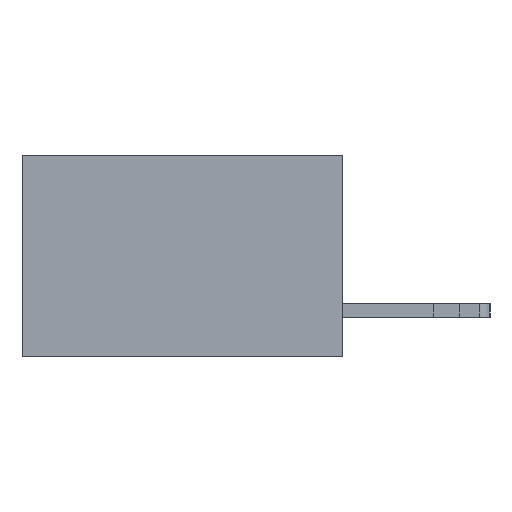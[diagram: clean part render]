
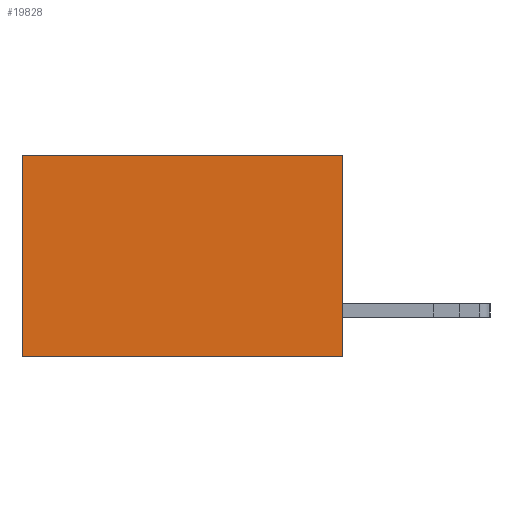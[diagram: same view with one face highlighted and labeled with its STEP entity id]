
A CAD part, left-side view. The second image highlights one B-rep face of the part: STEP entity #19828.
In plain terms, the highlighted planar face has unit normal (-1, 0, 0).
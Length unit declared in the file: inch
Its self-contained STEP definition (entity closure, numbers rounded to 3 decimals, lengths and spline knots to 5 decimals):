
#372 = VECTOR ( 'NONE', #17685, 39.37008 ) ;
#527 = EDGE_CURVE ( 'NONE', #11427, #15014, #13716, .T. ) ;
#1280 = DIRECTION ( 'NONE',  ( 0., 0., -1. ) ) ;
#1455 = CARTESIAN_POINT ( 'NONE',  ( 0.277, 0.59, -0.37 ) ) ;
#3148 = FACE_OUTER_BOUND ( 'NONE', #8072, .T. ) ;
#3642 = CARTESIAN_POINT ( 'NONE',  ( 0.277, 0., -0.37 ) ) ;
#3850 = ORIENTED_EDGE ( 'NONE', *, *, #6209, .F. ) ;
#4385 = CARTESIAN_POINT ( 'NONE',  ( 0.277, 0., 0. ) ) ;
#4778 = DIRECTION ( 'NONE',  ( 0., 0., -1. ) ) ;
#6189 = CARTESIAN_POINT ( 'NONE',  ( 0.277, 0., -0.37 ) ) ;
#6209 = EDGE_CURVE ( 'NONE', #8559, #17614, #8364, .T. ) ;
#6595 = CARTESIAN_POINT ( 'NONE',  ( 0.277, 0., -0.37 ) ) ;
#6766 = ORIENTED_EDGE ( 'NONE', *, *, #9300, .T. ) ;
#7045 = CARTESIAN_POINT ( 'NONE',  ( 0.277, 0., 0. ) ) ;
#7113 = VECTOR ( 'NONE', #8768, 39.37008 ) ;
#8072 = EDGE_LOOP ( 'NONE', ( #13944, #15072, #3850, #6766 ) ) ;
#8364 = LINE ( 'NONE', #6595, #12416 ) ;
#8559 = VERTEX_POINT ( 'NONE', #4385 ) ;
#8669 = CARTESIAN_POINT ( 'NONE',  ( 0.277, 0.59, -0.37 ) ) ;
#8768 = DIRECTION ( 'NONE',  ( 0., 1., 0. ) ) ;
#9300 = EDGE_CURVE ( 'NONE', #8559, #11427, #11163, .T. ) ;
#11163 = LINE ( 'NONE', #7045, #7113 ) ;
#11427 = VERTEX_POINT ( 'NONE', #17562 ) ;
#11622 = PLANE ( 'NONE',  #17821 ) ;
#12416 = VECTOR ( 'NONE', #1280, 39.37008 ) ;
#13359 = CARTESIAN_POINT ( 'NONE',  ( 0.277, 0., -0.37 ) ) ;
#13716 = LINE ( 'NONE', #1455, #372 ) ;
#13944 = ORIENTED_EDGE ( 'NONE', *, *, #527, .T. ) ;
#15014 = VERTEX_POINT ( 'NONE', #8669 ) ;
#15072 = ORIENTED_EDGE ( 'NONE', *, *, #15361, .F. ) ;
#15087 = DIRECTION ( 'NONE',  ( 1., 0., 0. ) ) ;
#15361 = EDGE_CURVE ( 'NONE', #17614, #15014, #16629, .T. ) ;
#16073 = VECTOR ( 'NONE', #19875, 39.37008 ) ;
#16629 = LINE ( 'NONE', #6189, #16073 ) ;
#17562 = CARTESIAN_POINT ( 'NONE',  ( 0.277, 0.59, 0. ) ) ;
#17614 = VERTEX_POINT ( 'NONE', #3642 ) ;
#17685 = DIRECTION ( 'NONE',  ( 0., 0., -1. ) ) ;
#17821 = AXIS2_PLACEMENT_3D ( 'NONE', #13359, #15087, #4778 ) ;
#19828 = ADVANCED_FACE ( 'NONE', ( #3148 ), #11622, .F. ) ;
#19875 = DIRECTION ( 'NONE',  ( 0., 1., 0. ) ) ;
